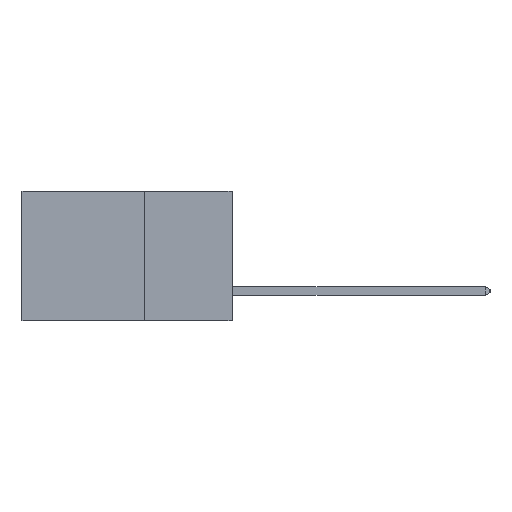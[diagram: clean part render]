
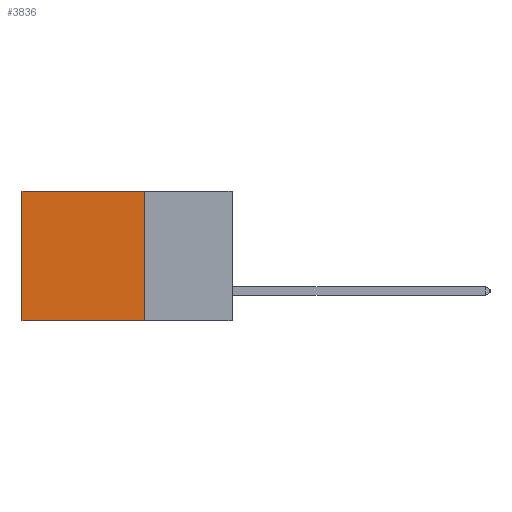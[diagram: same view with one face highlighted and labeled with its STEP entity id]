
A CAD part, left-side view. The second image highlights one B-rep face of the part: STEP entity #3836.
In plain terms, the highlighted planar face has unit normal (-1, 0, 0).
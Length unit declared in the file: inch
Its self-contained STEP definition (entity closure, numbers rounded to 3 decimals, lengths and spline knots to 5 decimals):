
#199 = VERTEX_POINT ( 'NONE', #1623 ) ;
#552 = VECTOR ( 'NONE', #15680, 39.37008 ) ;
#1623 = CARTESIAN_POINT ( 'NONE',  ( 0.2875, 0.6, -0.37 ) ) ;
#2046 = LINE ( 'NONE', #2503, #11411 ) ;
#2430 = DIRECTION ( 'NONE',  ( 0., 1., 0. ) ) ;
#2476 = EDGE_CURVE ( 'NONE', #18604, #199, #20610, .T. ) ;
#2503 = CARTESIAN_POINT ( 'NONE',  ( 0.2875, 0.25, -0.37 ) ) ;
#3405 = VERTEX_POINT ( 'NONE', #8946 ) ;
#3836 = ADVANCED_FACE ( 'NONE', ( #4700 ), #12755, .F. ) ;
#4170 = ORIENTED_EDGE ( 'NONE', *, *, #4191, .F. ) ;
#4191 = EDGE_CURVE ( 'NONE', #23987, #199, #2046, .T. ) ;
#4700 = FACE_OUTER_BOUND ( 'NONE', #21439, .T. ) ;
#5089 = EDGE_CURVE ( 'NONE', #3405, #23987, #19922, .T. ) ;
#5662 = VECTOR ( 'NONE', #15065, 39.37008 ) ;
#6741 = ORIENTED_EDGE ( 'NONE', *, *, #2476, .T. ) ;
#7083 = CARTESIAN_POINT ( 'NONE',  ( 0.2875, 0.25, -0.37 ) ) ;
#8946 = CARTESIAN_POINT ( 'NONE',  ( 0.2875, 0.25, 0. ) ) ;
#11411 = VECTOR ( 'NONE', #2430, 39.37008 ) ;
#11419 = CARTESIAN_POINT ( 'NONE',  ( 0.2875, 0.6, 0. ) ) ;
#12406 = DIRECTION ( 'NONE',  ( 0., 1., 0. ) ) ;
#12522 = DIRECTION ( 'NONE',  ( 0., 0., -1. ) ) ;
#12618 = DIRECTION ( 'NONE',  ( 1., 0., 0. ) ) ;
#12755 = PLANE ( 'NONE',  #18525 ) ;
#12791 = LINE ( 'NONE', #19972, #17184 ) ;
#12919 = CARTESIAN_POINT ( 'NONE',  ( 0.2875, 0.25, 0. ) ) ;
#14967 = CARTESIAN_POINT ( 'NONE',  ( 0.2875, 0.6, 0. ) ) ;
#15065 = DIRECTION ( 'NONE',  ( 0., 0., -1. ) ) ;
#15680 = DIRECTION ( 'NONE',  ( 0., 0., -1. ) ) ;
#16242 = CARTESIAN_POINT ( 'NONE',  ( 0.2875, 0.25, 0. ) ) ;
#17184 = VECTOR ( 'NONE', #12406, 39.37008 ) ;
#18312 = EDGE_CURVE ( 'NONE', #3405, #18604, #12791, .T. ) ;
#18525 = AXIS2_PLACEMENT_3D ( 'NONE', #12919, #12618, #12522 ) ;
#18604 = VERTEX_POINT ( 'NONE', #11419 ) ;
#19457 = ORIENTED_EDGE ( 'NONE', *, *, #18312, .T. ) ;
#19922 = LINE ( 'NONE', #16242, #552 ) ;
#19972 = CARTESIAN_POINT ( 'NONE',  ( 0.2875, 0.25, 0. ) ) ;
#20610 = LINE ( 'NONE', #14967, #5662 ) ;
#21439 = EDGE_LOOP ( 'NONE', ( #6741, #4170, #22210, #19457 ) ) ;
#22210 = ORIENTED_EDGE ( 'NONE', *, *, #5089, .F. ) ;
#23987 = VERTEX_POINT ( 'NONE', #7083 ) ;
